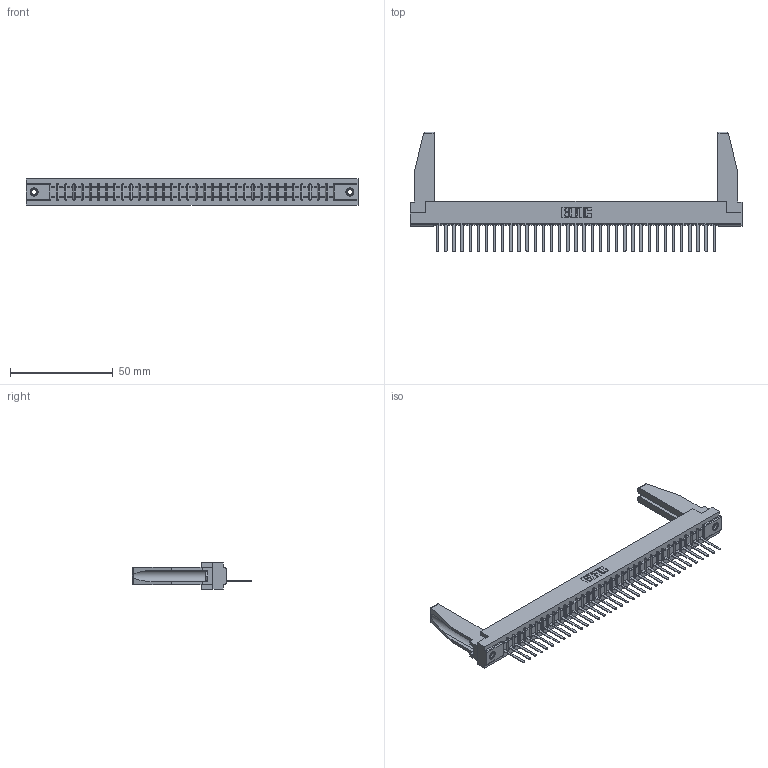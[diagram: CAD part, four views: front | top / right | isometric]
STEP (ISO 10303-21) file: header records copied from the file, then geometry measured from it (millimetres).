
FILE_DESCRIPTION (( 'STEP AP203' ), '1' );
FILE_NAME ('307-035-541-178.STEP', '2019-09-05T07:14:04', ( '' ), ( '' ), 'SwSTEP 2.0', 'SolidWorks 2016', '' );
FILE_SCHEMA (( 'CONFIG_CONTROL_DESIGN' ));
Length unit declared in the file: inch
Products named in the file (5): 307-220-078; 345-250-001_345-250-001-102; 307-035-541-178; 307-290-002_541; 307 Part_.156 Dia Mounting Holes
Assembly tree (40 placements, depth 2):
  307-035-541-178
    307 Part_.156 Dia Mounting Holes
    307-290-002_541  x35
    307-220-078  x2
    345-250-001_345-250-001-102  x2
Bounding box: 161.7 x 58.29 x 12.7 mm (x, y, z)
Volume: 21343.5 mm3; surface area: 26123 mm2
Topology: 40 solids, 40 shells, 2874 faces, 8773 edges, 5742 vertices
Faces by surface type: plane 1729, cylinder 1057, sphere 72, cone 12, torus 4
Entity records: 34025 total; most frequent: CARTESIAN_POINT 5738, ORIENTED_EDGE 5684, DIRECTION 5534, EDGE_CURVE 2842, VECTOR 2178, LINE 2178, VERTEX_POINT 1840, AXIS2_PLACEMENT_3D 1678
